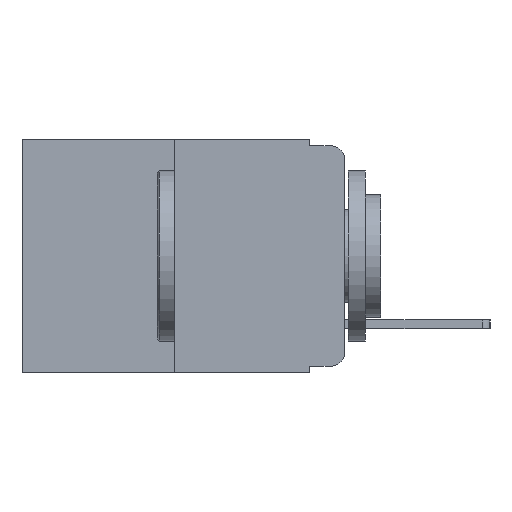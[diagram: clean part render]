
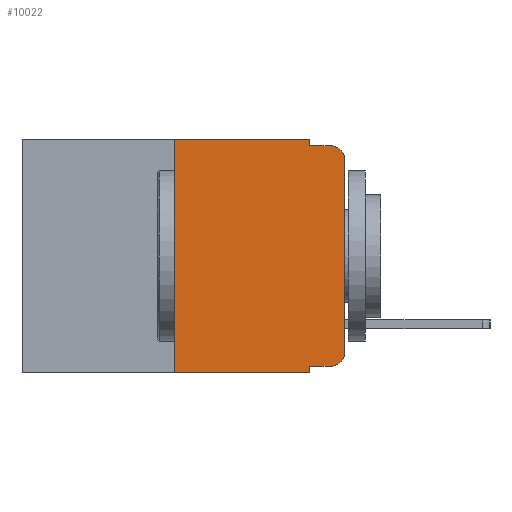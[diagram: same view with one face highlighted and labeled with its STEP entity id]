
A CAD part, left-side view. The second image highlights one B-rep face of the part: STEP entity #10022.
In plain terms, the highlighted planar face has unit normal (-1, 0, 0).
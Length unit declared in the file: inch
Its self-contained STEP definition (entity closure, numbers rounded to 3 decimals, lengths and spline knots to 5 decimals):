
#38 = VERTEX_POINT ( 'NONE', #4954 ) ;
#43 = DIRECTION ( 'NONE',  ( 0., -1., 0. ) ) ;
#189 = VERTEX_POINT ( 'NONE', #8098 ) ;
#826 = FACE_OUTER_BOUND ( 'NONE', #9310, .T. ) ;
#916 = EDGE_CURVE ( 'NONE', #2093, #5427, #6904, .T. ) ;
#1062 = ORIENTED_EDGE ( 'NONE', *, *, #9618, .F. ) ;
#1119 = VERTEX_POINT ( 'NONE', #2890 ) ;
#1618 = CARTESIAN_POINT ( 'NONE',  ( 0., 0.02, -0.313 ) ) ;
#1912 = CARTESIAN_POINT ( 'NONE',  ( 0., 0.25, -0.343 ) ) ;
#2093 = VERTEX_POINT ( 'NONE', #10991 ) ;
#2333 = CARTESIAN_POINT ( 'NONE',  ( 0., 0.02, -0.01 ) ) ;
#2642 = CARTESIAN_POINT ( 'NONE',  ( 0., 0.051, 0. ) ) ;
#2681 = DIRECTION ( 'NONE',  ( 0., 0., -1. ) ) ;
#2728 = LINE ( 'NONE', #2918, #12313 ) ;
#2890 = CARTESIAN_POINT ( 'NONE',  ( 0., 0., -0.313 ) ) ;
#2897 = VERTEX_POINT ( 'NONE', #1912 ) ;
#2918 = CARTESIAN_POINT ( 'NONE',  ( 0., 0.473, -0.343 ) ) ;
#3061 = EDGE_CURVE ( 'NONE', #5427, #6947, #4566, .T. ) ;
#3202 = VECTOR ( 'NONE', #11099, 39.37008 ) ;
#3308 = EDGE_CURVE ( 'NONE', #11862, #1119, #11507, .T. ) ;
#3388 = CARTESIAN_POINT ( 'NONE',  ( 0., 0.02, -0.03 ) ) ;
#3567 = CARTESIAN_POINT ( 'NONE',  ( 0., 0.02, -0.333 ) ) ;
#3644 = CARTESIAN_POINT ( 'NONE',  ( 0., 0.473, 0. ) ) ;
#3722 = AXIS2_PLACEMENT_3D ( 'NONE', #1618, #8394, #2681 ) ;
#3797 = VERTEX_POINT ( 'NONE', #7292 ) ;
#4082 = EDGE_CURVE ( 'NONE', #2897, #3797, #2728, .T. ) ;
#4339 = DIRECTION ( 'NONE',  ( 0., 0., -1. ) ) ;
#4344 = EDGE_CURVE ( 'NONE', #10930, #2093, #5480, .T. ) ;
#4566 = LINE ( 'NONE', #6158, #8987 ) ;
#4594 = DIRECTION ( 'NONE',  ( 0., 0., -1. ) ) ;
#4617 = VECTOR ( 'NONE', #11968, 39.37008 ) ;
#4950 = DIRECTION ( 'NONE',  ( 0., 0., 1. ) ) ;
#4954 = CARTESIAN_POINT ( 'NONE',  ( 0., 0.051, -0.333 ) ) ;
#5140 = DIRECTION ( 'NONE',  ( 0., 0., -1. ) ) ;
#5427 = VERTEX_POINT ( 'NONE', #7716 ) ;
#5480 = LINE ( 'NONE', #5604, #3202 ) ;
#5604 = CARTESIAN_POINT ( 'NONE',  ( 0., 0.473, 0. ) ) ;
#5683 = EDGE_CURVE ( 'NONE', #189, #6947, #7405, .T. ) ;
#6158 = CARTESIAN_POINT ( 'NONE',  ( 0., 0.051, -0.01 ) ) ;
#6412 = ORIENTED_EDGE ( 'NONE', *, *, #9999, .T. ) ;
#6426 = LINE ( 'NONE', #7826, #11243 ) ;
#6567 = ORIENTED_EDGE ( 'NONE', *, *, #3061, .F. ) ;
#6572 = EDGE_CURVE ( 'NONE', #38, #11862, #10062, .T. ) ;
#6687 = CARTESIAN_POINT ( 'NONE',  ( 0., 0.051, -0.333 ) ) ;
#6904 = LINE ( 'NONE', #8575, #11686 ) ;
#6947 = VERTEX_POINT ( 'NONE', #2333 ) ;
#7015 = ORIENTED_EDGE ( 'NONE', *, *, #4082, .T. ) ;
#7204 = LINE ( 'NONE', #2642, #4617 ) ;
#7292 = CARTESIAN_POINT ( 'NONE',  ( 0., 0.051, -0.343 ) ) ;
#7405 = CIRCLE ( 'NONE', #8349, 0.02 ) ;
#7589 = ORIENTED_EDGE ( 'NONE', *, *, #7806, .F. ) ;
#7716 = CARTESIAN_POINT ( 'NONE',  ( 0., 0.051, -0.01 ) ) ;
#7806 = EDGE_CURVE ( 'NONE', #38, #3797, #7204, .T. ) ;
#7826 = CARTESIAN_POINT ( 'NONE',  ( 0., 0.25, 0. ) ) ;
#7865 = ORIENTED_EDGE ( 'NONE', *, *, #6572, .T. ) ;
#8098 = CARTESIAN_POINT ( 'NONE',  ( 0., 0., -0.03 ) ) ;
#8349 = AXIS2_PLACEMENT_3D ( 'NONE', #3388, #9953, #4339 ) ;
#8394 = DIRECTION ( 'NONE',  ( -1., 0., 0. ) ) ;
#8575 = CARTESIAN_POINT ( 'NONE',  ( 0., 0.051, 0. ) ) ;
#8926 = VECTOR ( 'NONE', #10114, 39.37008 ) ;
#8938 = CARTESIAN_POINT ( 'NONE',  ( 0., 0.25, 0. ) ) ;
#8987 = VECTOR ( 'NONE', #43, 39.37008 ) ;
#9286 = PLANE ( 'NONE',  #11315 ) ;
#9310 = EDGE_LOOP ( 'NONE', ( #6412, #10534, #6567, #11657, #11920, #1062, #7015, #7589, #7865, #10547 ) ) ;
#9618 = EDGE_CURVE ( 'NONE', #2897, #10930, #6426, .T. ) ;
#9777 = VECTOR ( 'NONE', #12064, 39.37008 ) ;
#9953 = DIRECTION ( 'NONE',  ( -1., 0., 0. ) ) ;
#9999 = EDGE_CURVE ( 'NONE', #1119, #189, #11047, .T. ) ;
#10022 = ADVANCED_FACE ( 'NONE', ( #826 ), #9286, .F. ) ;
#10062 = LINE ( 'NONE', #6687, #9777 ) ;
#10114 = DIRECTION ( 'NONE',  ( 0., 0., 1. ) ) ;
#10154 = CARTESIAN_POINT ( 'NONE',  ( 0., 0., 0. ) ) ;
#10196 = DIRECTION ( 'NONE',  ( 1., 0., 0. ) ) ;
#10534 = ORIENTED_EDGE ( 'NONE', *, *, #5683, .T. ) ;
#10547 = ORIENTED_EDGE ( 'NONE', *, *, #3308, .T. ) ;
#10930 = VERTEX_POINT ( 'NONE', #8938 ) ;
#10991 = CARTESIAN_POINT ( 'NONE',  ( 0., 0.051, 0. ) ) ;
#11047 = LINE ( 'NONE', #10154, #8926 ) ;
#11099 = DIRECTION ( 'NONE',  ( 0., -1., 0. ) ) ;
#11243 = VECTOR ( 'NONE', #4950, 39.37008 ) ;
#11315 = AXIS2_PLACEMENT_3D ( 'NONE', #3644, #10196, #4594 ) ;
#11507 = CIRCLE ( 'NONE', #3722, 0.02 ) ;
#11657 = ORIENTED_EDGE ( 'NONE', *, *, #916, .F. ) ;
#11686 = VECTOR ( 'NONE', #5140, 39.37008 ) ;
#11862 = VERTEX_POINT ( 'NONE', #3567 ) ;
#11920 = ORIENTED_EDGE ( 'NONE', *, *, #4344, .F. ) ;
#11968 = DIRECTION ( 'NONE',  ( 0., 0., -1. ) ) ;
#12064 = DIRECTION ( 'NONE',  ( 0., -1., 0. ) ) ;
#12210 = DIRECTION ( 'NONE',  ( 0., -1., 0. ) ) ;
#12313 = VECTOR ( 'NONE', #12210, 39.37008 ) ;
